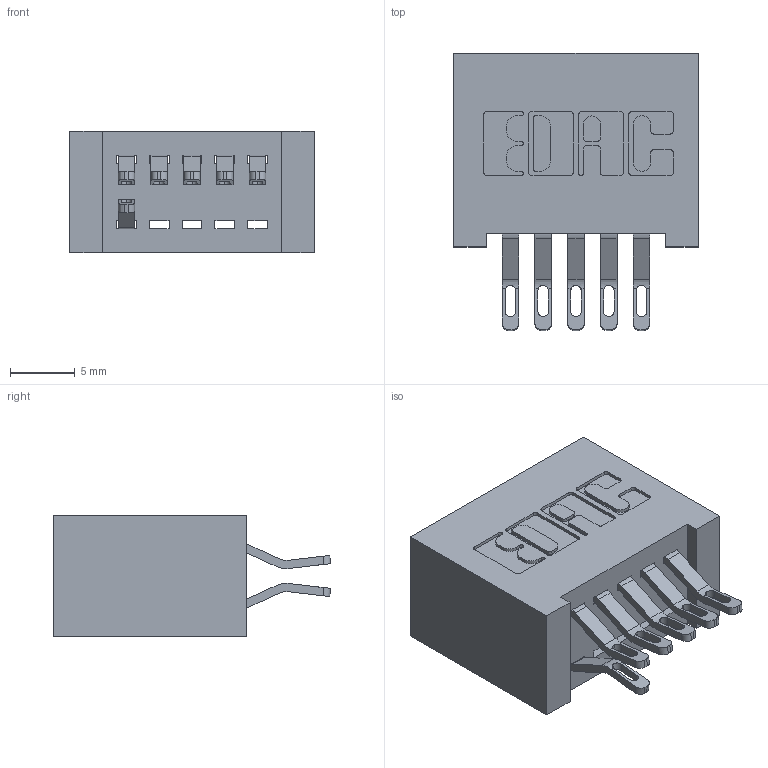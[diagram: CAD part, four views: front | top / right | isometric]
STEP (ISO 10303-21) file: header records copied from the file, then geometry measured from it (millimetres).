
FILE_DESCRIPTION (( 'STEP AP203' ), '1' );
FILE_NAME ('392-010-555-201.STEP', '2018-08-14T20:47:09', ( '' ), ( '' ), 'SwSTEP 2.0', 'SolidWorks 2016', '' );
FILE_SCHEMA (( 'CONFIG_CONTROL_DESIGN' ));
Length unit declared in the file: inch
Products named in the file (3): 342 Part_Lugless; 345-292-001_555 Tail; 392-010-555-201
Assembly tree (7 placements, depth 2):
  392-010-555-201
    342 Part_Lugless
    345-292-001_555 Tail  x6
Bounding box: 18.95 x 21.47 x 9.4 mm (x, y, z)
Volume: 1947.6 mm3; surface area: 2563.8 mm2
Topology: 7 solids, 7 shells, 474 faces, 1457 edges, 970 vertices
Faces by surface type: plane 290, cylinder 184
Entity records: 7791 total; most frequent: CARTESIAN_POINT 1384, ORIENTED_EDGE 1294, DIRECTION 1207, EDGE_CURVE 647, LINE 507, VECTOR 507, VERTEX_POINT 430, AXIS2_PLACEMENT_3D 350
